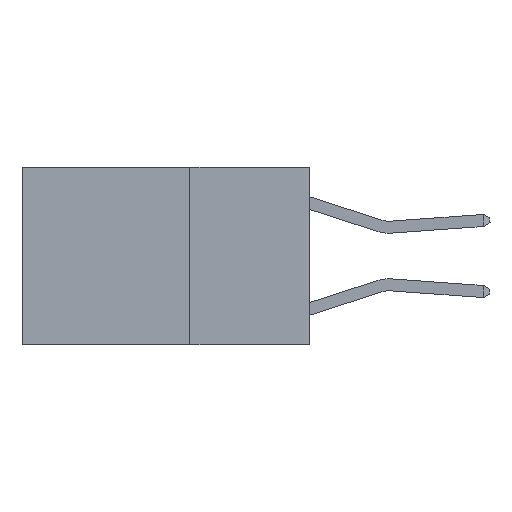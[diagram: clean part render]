
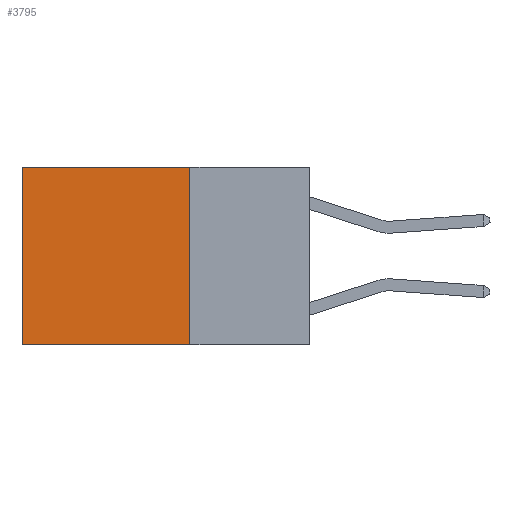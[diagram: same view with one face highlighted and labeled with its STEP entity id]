
A CAD part, left-side view. The second image highlights one B-rep face of the part: STEP entity #3795.
In plain terms, the highlighted planar face has unit normal (-1, 0, 0).
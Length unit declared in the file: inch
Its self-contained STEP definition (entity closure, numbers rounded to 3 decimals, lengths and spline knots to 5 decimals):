
#93 = PLANE ( 'NONE',  #7777 ) ;
#129 = LINE ( 'NONE', #9999, #2410 ) ;
#260 = ORIENTED_EDGE ( 'NONE', *, *, #8602, .F. ) ;
#347 = DIRECTION ( 'NONE',  ( 0., 1., 0. ) ) ;
#894 = LINE ( 'NONE', #7128, #7997 ) ;
#901 = DIRECTION ( 'NONE',  ( 0., 0., -1. ) ) ;
#1098 = DIRECTION ( 'NONE',  ( 1., 0., 0. ) ) ;
#1675 = VECTOR ( 'NONE', #901, 39.37008 ) ;
#2410 = VECTOR ( 'NONE', #8087, 39.37008 ) ;
#2529 = ORIENTED_EDGE ( 'NONE', *, *, #6754, .T. ) ;
#2938 = EDGE_CURVE ( 'NONE', #3733, #6306, #11804, .T. ) ;
#2948 = VERTEX_POINT ( 'NONE', #11426 ) ;
#2988 = FACE_OUTER_BOUND ( 'NONE', #5846, .T. ) ;
#3219 = CARTESIAN_POINT ( 'NONE',  ( 0.2625, 0.6, 0. ) ) ;
#3442 = ORIENTED_EDGE ( 'NONE', *, *, #2938, .F. ) ;
#3733 = VERTEX_POINT ( 'NONE', #11409 ) ;
#3795 = ADVANCED_FACE ( 'NONE', ( #2988 ), #93, .F. ) ;
#3929 = EDGE_CURVE ( 'NONE', #3733, #8998, #894, .T. ) ;
#4447 = DIRECTION ( 'NONE',  ( 0., 0., -1. ) ) ;
#5846 = EDGE_LOOP ( 'NONE', ( #2529, #260, #3442, #8606 ) ) ;
#6306 = VERTEX_POINT ( 'NONE', #9559 ) ;
#6691 = CARTESIAN_POINT ( 'NONE',  ( 0.2625, 0.25, 0. ) ) ;
#6754 = EDGE_CURVE ( 'NONE', #8998, #2948, #8213, .T. ) ;
#6889 = CARTESIAN_POINT ( 'NONE',  ( 0.2625, 0.25, 0. ) ) ;
#7128 = CARTESIAN_POINT ( 'NONE',  ( 0.2625, 0.25, 0. ) ) ;
#7777 = AXIS2_PLACEMENT_3D ( 'NONE', #6889, #1098, #7840 ) ;
#7840 = DIRECTION ( 'NONE',  ( 0., 0., -1. ) ) ;
#7913 = VECTOR ( 'NONE', #4447, 39.37008 ) ;
#7997 = VECTOR ( 'NONE', #347, 39.37008 ) ;
#8087 = DIRECTION ( 'NONE',  ( 0., 1., 0. ) ) ;
#8213 = LINE ( 'NONE', #8371, #7913 ) ;
#8371 = CARTESIAN_POINT ( 'NONE',  ( 0.2625, 0.6, 0. ) ) ;
#8602 = EDGE_CURVE ( 'NONE', #6306, #2948, #129, .T. ) ;
#8606 = ORIENTED_EDGE ( 'NONE', *, *, #3929, .T. ) ;
#8998 = VERTEX_POINT ( 'NONE', #3219 ) ;
#9559 = CARTESIAN_POINT ( 'NONE',  ( 0.2625, 0.25, -0.37 ) ) ;
#9999 = CARTESIAN_POINT ( 'NONE',  ( 0.2625, 0.25, -0.37 ) ) ;
#11409 = CARTESIAN_POINT ( 'NONE',  ( 0.2625, 0.25, 0. ) ) ;
#11426 = CARTESIAN_POINT ( 'NONE',  ( 0.2625, 0.6, -0.37 ) ) ;
#11804 = LINE ( 'NONE', #6691, #1675 ) ;
